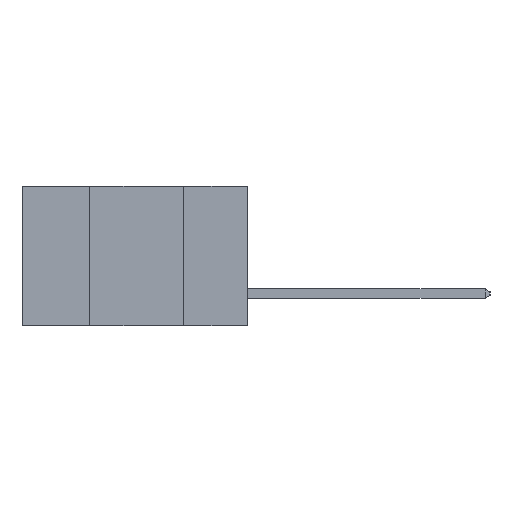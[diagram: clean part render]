
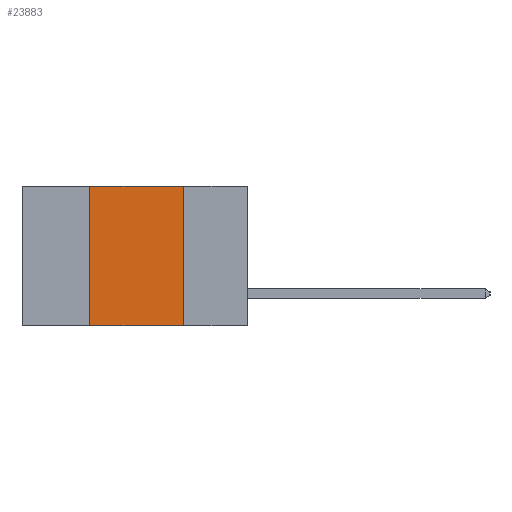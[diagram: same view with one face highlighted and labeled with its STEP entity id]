
A CAD part, left-side view. The second image highlights one B-rep face of the part: STEP entity #23883.
In plain terms, the highlighted planar face has unit normal (-1, 0, 0).
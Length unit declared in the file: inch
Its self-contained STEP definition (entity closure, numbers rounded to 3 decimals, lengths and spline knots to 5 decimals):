
#2070 = PLANE ( 'NONE',  #20634 ) ;
#2140 = VERTEX_POINT ( 'NONE', #20454 ) ;
#2910 = EDGE_CURVE ( 'NONE', #13228, #2140, #23557, .T. ) ;
#3190 = EDGE_CURVE ( 'NONE', #2140, #13364, #15902, .T. ) ;
#3429 = CARTESIAN_POINT ( 'NONE',  ( 0., 0.6, 0. ) ) ;
#3875 = DIRECTION ( 'NONE',  ( 0., -1., 0. ) ) ;
#4309 = CARTESIAN_POINT ( 'NONE',  ( 0., 0.42, 0. ) ) ;
#6194 = DIRECTION ( 'NONE',  ( 0., 0., -1. ) ) ;
#6894 = VECTOR ( 'NONE', #22755, 39.37008 ) ;
#7276 = EDGE_CURVE ( 'NONE', #17906, #13364, #7938, .T. ) ;
#7938 = LINE ( 'NONE', #23035, #18249 ) ;
#8900 = ORIENTED_EDGE ( 'NONE', *, *, #3190, .F. ) ;
#12758 = VECTOR ( 'NONE', #3875, 39.37008 ) ;
#13228 = VERTEX_POINT ( 'NONE', #4309 ) ;
#13364 = VERTEX_POINT ( 'NONE', #19107 ) ;
#14187 = EDGE_CURVE ( 'NONE', #17906, #13228, #23216, .T. ) ;
#14902 = ORIENTED_EDGE ( 'NONE', *, *, #7276, .T. ) ;
#15007 = ORIENTED_EDGE ( 'NONE', *, *, #14187, .F. ) ;
#15274 = VECTOR ( 'NONE', #23378, 39.37008 ) ;
#15379 = FACE_OUTER_BOUND ( 'NONE', #15640, .T. ) ;
#15640 = EDGE_LOOP ( 'NONE', ( #8900, #23792, #15007, #14902 ) ) ;
#15902 = LINE ( 'NONE', #23463, #15274 ) ;
#16444 = CARTESIAN_POINT ( 'NONE',  ( 0., 0.6, 0. ) ) ;
#17906 = VERTEX_POINT ( 'NONE', #22739 ) ;
#18249 = VECTOR ( 'NONE', #25028, 39.37008 ) ;
#18508 = DIRECTION ( 'NONE',  ( 1., 0., 0. ) ) ;
#19107 = CARTESIAN_POINT ( 'NONE',  ( 0., 0.17, -0.37 ) ) ;
#20454 = CARTESIAN_POINT ( 'NONE',  ( 0., 0.17, 0. ) ) ;
#20634 = AXIS2_PLACEMENT_3D ( 'NONE', #16444, #18508, #6194 ) ;
#20696 = CARTESIAN_POINT ( 'NONE',  ( 0., 0.42, 0. ) ) ;
#22739 = CARTESIAN_POINT ( 'NONE',  ( 0., 0.42, -0.37 ) ) ;
#22755 = DIRECTION ( 'NONE',  ( 0., 0., 1. ) ) ;
#23035 = CARTESIAN_POINT ( 'NONE',  ( 0., 0.6, -0.37 ) ) ;
#23216 = LINE ( 'NONE', #20696, #6894 ) ;
#23378 = DIRECTION ( 'NONE',  ( 0., 0., -1. ) ) ;
#23463 = CARTESIAN_POINT ( 'NONE',  ( 0., 0.17, 0. ) ) ;
#23557 = LINE ( 'NONE', #3429, #12758 ) ;
#23792 = ORIENTED_EDGE ( 'NONE', *, *, #2910, .F. ) ;
#23883 = ADVANCED_FACE ( 'NONE', ( #15379 ), #2070, .F. ) ;
#25028 = DIRECTION ( 'NONE',  ( 0., -1., 0. ) ) ;
